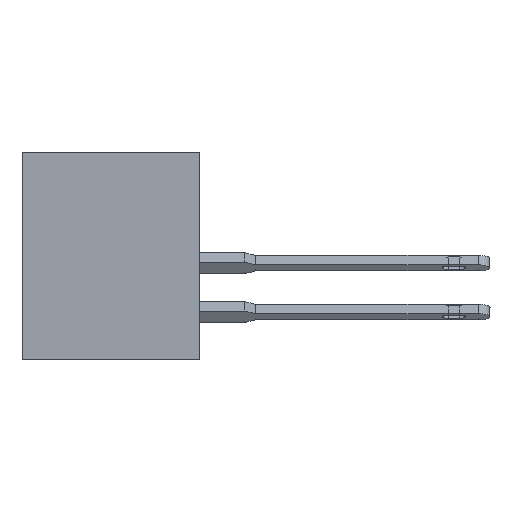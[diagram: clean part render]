
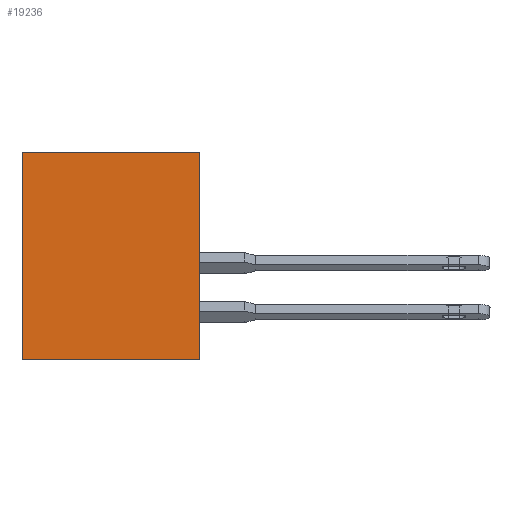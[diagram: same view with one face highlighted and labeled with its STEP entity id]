
A CAD part, left-side view. The second image highlights one B-rep face of the part: STEP entity #19236.
In plain terms, the highlighted planar face has unit normal (-1, 0, 0).
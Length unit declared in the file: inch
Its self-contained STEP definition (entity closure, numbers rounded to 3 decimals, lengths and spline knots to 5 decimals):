
#363 = LINE ( 'NONE', #23778, #19674 ) ;
#984 = EDGE_LOOP ( 'NONE', ( #18571, #24667, #24347, #12367 ) ) ;
#1980 = DIRECTION ( 'NONE',  ( 0., 0., 1. ) ) ;
#2720 = PLANE ( 'NONE',  #23885 ) ;
#4664 = CARTESIAN_POINT ( 'NONE',  ( 0., 0.453, 0. ) ) ;
#5245 = EDGE_CURVE ( 'NONE', #16027, #6200, #24485, .T. ) ;
#5665 = CARTESIAN_POINT ( 'NONE',  ( 0., 0., 0. ) ) ;
#6150 = EDGE_CURVE ( 'NONE', #14189, #6200, #7098, .T. ) ;
#6200 = VERTEX_POINT ( 'NONE', #5665 ) ;
#6721 = CARTESIAN_POINT ( 'NONE',  ( 0., 0., -0.531 ) ) ;
#7098 = LINE ( 'NONE', #8084, #19642 ) ;
#7147 = VECTOR ( 'NONE', #1980, 39.37008 ) ;
#8084 = CARTESIAN_POINT ( 'NONE',  ( 0., 0.453, 0. ) ) ;
#10040 = FACE_OUTER_BOUND ( 'NONE', #984, .T. ) ;
#12367 = ORIENTED_EDGE ( 'NONE', *, *, #19911, .T. ) ;
#14125 = VERTEX_POINT ( 'NONE', #24807 ) ;
#14189 = VERTEX_POINT ( 'NONE', #4664 ) ;
#14594 = CARTESIAN_POINT ( 'NONE',  ( 0., 0., 0. ) ) ;
#16027 = VERTEX_POINT ( 'NONE', #6721 ) ;
#16306 = VECTOR ( 'NONE', #19425, 39.37008 ) ;
#17159 = CARTESIAN_POINT ( 'NONE',  ( 0., 0.453, 0. ) ) ;
#17488 = DIRECTION ( 'NONE',  ( 0., -1., 0. ) ) ;
#18556 = DIRECTION ( 'NONE',  ( 1., 0., 0. ) ) ;
#18571 = ORIENTED_EDGE ( 'NONE', *, *, #5245, .T. ) ;
#19236 = ADVANCED_FACE ( 'NONE', ( #10040 ), #2720, .F. ) ;
#19425 = DIRECTION ( 'NONE',  ( 0., 0., 1. ) ) ;
#19642 = VECTOR ( 'NONE', #26323, 39.37008 ) ;
#19674 = VECTOR ( 'NONE', #17488, 39.37008 ) ;
#19858 = EDGE_CURVE ( 'NONE', #14125, #14189, #26283, .T. ) ;
#19911 = EDGE_CURVE ( 'NONE', #14125, #16027, #363, .T. ) ;
#22727 = CARTESIAN_POINT ( 'NONE',  ( 0., 0.453, 0. ) ) ;
#23778 = CARTESIAN_POINT ( 'NONE',  ( 0., 0.453, -0.531 ) ) ;
#23885 = AXIS2_PLACEMENT_3D ( 'NONE', #22727, #18556, #25210 ) ;
#24347 = ORIENTED_EDGE ( 'NONE', *, *, #19858, .F. ) ;
#24485 = LINE ( 'NONE', #14594, #7147 ) ;
#24667 = ORIENTED_EDGE ( 'NONE', *, *, #6150, .F. ) ;
#24807 = CARTESIAN_POINT ( 'NONE',  ( 0., 0.453, -0.531 ) ) ;
#25210 = DIRECTION ( 'NONE',  ( 0., 0., -1. ) ) ;
#26283 = LINE ( 'NONE', #17159, #16306 ) ;
#26323 = DIRECTION ( 'NONE',  ( 0., -1., 0. ) ) ;
